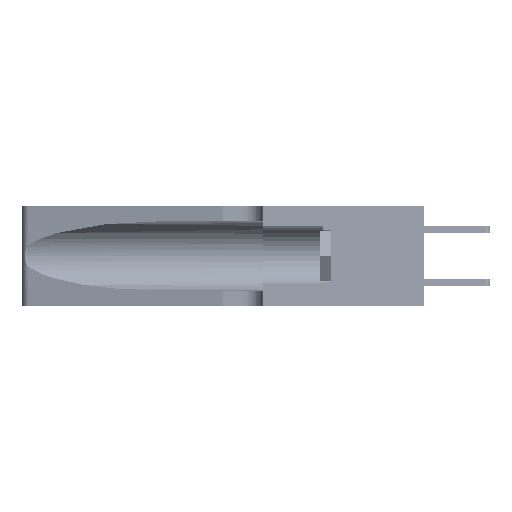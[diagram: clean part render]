
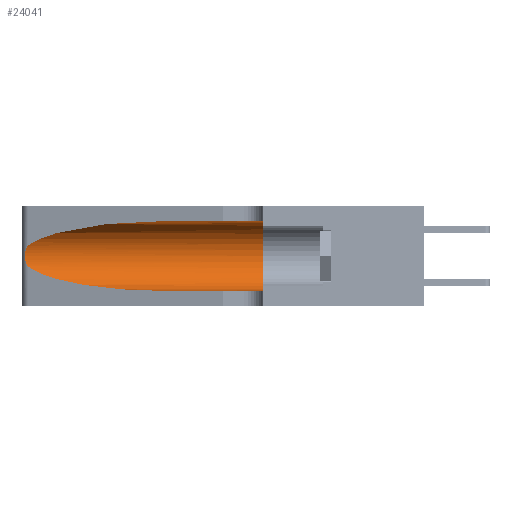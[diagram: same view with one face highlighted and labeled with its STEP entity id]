
A CAD part, left-side view. The second image highlights one B-rep face of the part: STEP entity #24041.
In plain terms, the highlighted cylindrical face has radius 3.308 mm (diameter 6.617 mm), a partial arc.
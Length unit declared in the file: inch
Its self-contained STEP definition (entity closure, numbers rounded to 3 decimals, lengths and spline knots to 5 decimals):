
#3039 = VERTEX_POINT ( 'NONE', #38732 ) ;
#3671 = CARTESIAN_POINT ( 'NONE',  ( 0.26075, 1.23896, 0.178 ) ) ;
#3803 = ORIENTED_EDGE ( 'NONE', *, *, #37399, .T. ) ;
#5293 = CARTESIAN_POINT ( 'NONE',  ( 0.1305, 0.35, 0.31525 ) ) ;
#6986 = B_SPLINE_CURVE_WITH_KNOTS ( 'NONE', 3,
 ( #14668, #11167, #37877, #33537, #10663, #41385, #37393, #3671, #49193, #48852, #15000, #18494, #45208, #26157 ),
 .UNSPECIFIED., .F., .F.,
 ( 4, 2, 2, 2, 2, 2, 4 ),
 ( 0., 0.00027, 0.00053, 0.00107, 0.0016, 0.00187, 0.00214 ),
 .UNSPECIFIED. ) ;
#7660 = LINE ( 'NONE', #19330, #32769 ) ;
#7771 = VERTEX_POINT ( 'NONE', #5293 ) ;
#7978 = DIRECTION ( 'NONE',  ( 0., -1., 0. ) ) ;
#10282 = DIRECTION ( 'NONE',  ( 0., 1., 0. ) ) ;
#10654 =( BOUNDED_CURVE ( )  B_SPLINE_CURVE ( 3, ( #12611, #24441, #47962, #32293 ),
 .UNSPECIFIED., .F., .T. ) 
 B_SPLINE_CURVE_WITH_KNOTS ( ( 4, 4 ),
 ( 3.44316, 4.71239 ),
 .UNSPECIFIED. ) 
 CURVE ( )  GEOMETRIC_REPRESENTATION_ITEM ( )  RATIONAL_B_SPLINE_CURVE ( ( 1., 0.87, 0.87, 1. ) ) 
 REPRESENTATION_ITEM ( '' )  );
#10663 = CARTESIAN_POINT ( 'NONE',  ( 0.25854, 1.2359, 0.20912 ) ) ;
#10748 = DIRECTION ( 'NONE',  ( 0., 0., -1. ) ) ;
#10907 = VERTEX_POINT ( 'NONE', #13864 ) ;
#11167 = CARTESIAN_POINT ( 'NONE',  ( 0.25555, 1.22994, 0.2215 ) ) ;
#11563 = DIRECTION ( 'NONE',  ( 0., -1., 0. ) ) ;
#12186 = VECTOR ( 'NONE', #11563, 39.37008 ) ;
#12531 = EDGE_LOOP ( 'NONE', ( #30380, #41447, #30930, #3803, #31685, #31670 ) ) ;
#12611 = CARTESIAN_POINT ( 'NONE',  ( 0.25487, 1.22718, 0.14631 ) ) ;
#13227 = EDGE_CURVE ( 'NONE', #41033, #10907, #6986, .T. ) ;
#13297 = EDGE_CURVE ( 'NONE', #27430, #7771, #7660, .T. ) ;
#13864 = CARTESIAN_POINT ( 'NONE',  ( 0.25487, 1.22718, 0.14631 ) ) ;
#14668 = CARTESIAN_POINT ( 'NONE',  ( 0.25487, 1.22718, 0.22369 ) ) ;
#15000 = CARTESIAN_POINT ( 'NONE',  ( 0.25789, 1.23486, 0.15765 ) ) ;
#17773 = CARTESIAN_POINT ( 'NONE',  ( 0.18966, 0.96281, 0.31525 ) ) ;
#18494 = CARTESIAN_POINT ( 'NONE',  ( 0.25639, 1.23186, 0.15144 ) ) ;
#19330 = CARTESIAN_POINT ( 'NONE',  ( 0.1305, 1.61858, 0.31525 ) ) ;
#21775 = DIRECTION ( 'NONE',  ( 0., -1., 0. ) ) ;
#21782 = CARTESIAN_POINT ( 'NONE',  ( 0.2373, 1.15595, 0.28018 ) ) ;
#24041 = ADVANCED_FACE ( 'NONE', ( #45150 ), #48114, .F. ) ;
#24441 = CARTESIAN_POINT ( 'NONE',  ( 0.2373, 1.15595, 0.08982 ) ) ;
#26157 = CARTESIAN_POINT ( 'NONE',  ( 0.25487, 1.22718, 0.14631 ) ) ;
#26413 = CARTESIAN_POINT ( 'NONE',  ( 0.25487, 1.22718, 0.22369 ) ) ;
#27430 = VERTEX_POINT ( 'NONE', #48607 ) ;
#28281 = LINE ( 'NONE', #38266, #12186 ) ;
#30380 = ORIENTED_EDGE ( 'NONE', *, *, #42658, .T. ) ;
#30688 = EDGE_CURVE ( 'NONE', #10907, #3039, #10654, .T. ) ;
#30930 = ORIENTED_EDGE ( 'NONE', *, *, #30688, .T. ) ;
#31670 = ORIENTED_EDGE ( 'NONE', *, *, #13297, .F. ) ;
#31685 = ORIENTED_EDGE ( 'NONE', *, *, #48436, .F. ) ;
#32293 = CARTESIAN_POINT ( 'NONE',  ( 0.1305, 0.72297, 0.05475 ) ) ;
#32769 = VECTOR ( 'NONE', #7978, 39.37008 ) ;
#33324 = DIRECTION ( 'NONE',  ( 0., 0., 1. ) ) ;
#33537 = CARTESIAN_POINT ( 'NONE',  ( 0.25787, 1.23484, 0.2124 ) ) ;
#33569 = AXIS2_PLACEMENT_3D ( 'NONE', #44493, #10282, #33324 ) ;
#33862 = AXIS2_PLACEMENT_3D ( 'NONE', #45285, #21775, #10748 ) ;
#33968 = VERTEX_POINT ( 'NONE', #47710 ) ;
#34090 = CARTESIAN_POINT ( 'NONE',  ( 0.25487, 1.22718, 0.22369 ) ) ;
#37393 = CARTESIAN_POINT ( 'NONE',  ( 0.26075, 1.23896, 0.19203 ) ) ;
#37399 = EDGE_CURVE ( 'NONE', #3039, #33968, #28281, .T. ) ;
#37877 = CARTESIAN_POINT ( 'NONE',  ( 0.25639, 1.23184, 0.21858 ) ) ;
#38266 = CARTESIAN_POINT ( 'NONE',  ( 0.1305, 1.61858, 0.05475 ) ) ;
#38732 = CARTESIAN_POINT ( 'NONE',  ( 0.1305, 0.72297, 0.05475 ) ) ;
#41033 = VERTEX_POINT ( 'NONE', #34090 ) ;
#41385 = CARTESIAN_POINT ( 'NONE',  ( 0.26018, 1.23835, 0.19895 ) ) ;
#41447 = ORIENTED_EDGE ( 'NONE', *, *, #13227, .T. ) ;
#42658 = EDGE_CURVE ( 'NONE', #27430, #41033, #43391, .T. ) ;
#43391 =( BOUNDED_CURVE ( )  B_SPLINE_CURVE ( 3, ( #48786, #17773, #21782, #26413 ),
 .UNSPECIFIED., .F., .T. ) 
 B_SPLINE_CURVE_WITH_KNOTS ( ( 4, 4 ),
 ( 1.5708, 2.84003 ),
 .UNSPECIFIED. ) 
 CURVE ( )  GEOMETRIC_REPRESENTATION_ITEM ( )  RATIONAL_B_SPLINE_CURVE ( ( 1., 0.87, 0.87, 1. ) ) 
 REPRESENTATION_ITEM ( '' )  );
#44493 = CARTESIAN_POINT ( 'NONE',  ( 0.1305, 0.35, 0.185 ) ) ;
#45150 = FACE_OUTER_BOUND ( 'NONE', #12531, .T. ) ;
#45208 = CARTESIAN_POINT ( 'NONE',  ( 0.25555, 1.22993, 0.14849 ) ) ;
#45285 = CARTESIAN_POINT ( 'NONE',  ( 0.1305, 1.61858, 0.185 ) ) ;
#47710 = CARTESIAN_POINT ( 'NONE',  ( 0.1305, 0.35, 0.05475 ) ) ;
#47962 = CARTESIAN_POINT ( 'NONE',  ( 0.18966, 0.96281, 0.05475 ) ) ;
#48114 = CYLINDRICAL_SURFACE ( 'NONE', #33862, 0.13025 ) ;
#48275 = CIRCLE ( 'NONE', #33569, 0.13025 ) ;
#48436 = EDGE_CURVE ( 'NONE', #7771, #33968, #48275, .T. ) ;
#48607 = CARTESIAN_POINT ( 'NONE',  ( 0.1305, 0.72297, 0.31525 ) ) ;
#48786 = CARTESIAN_POINT ( 'NONE',  ( 0.1305, 0.72297, 0.31525 ) ) ;
#48852 = CARTESIAN_POINT ( 'NONE',  ( 0.25856, 1.23593, 0.16098 ) ) ;
#49193 = CARTESIAN_POINT ( 'NONE',  ( 0.26017, 1.23833, 0.17102 ) ) ;
